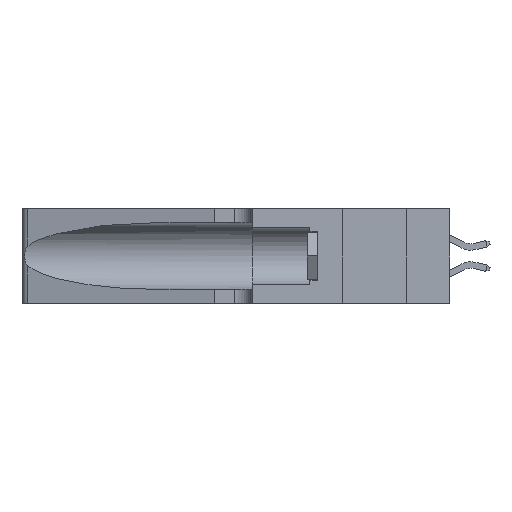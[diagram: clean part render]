
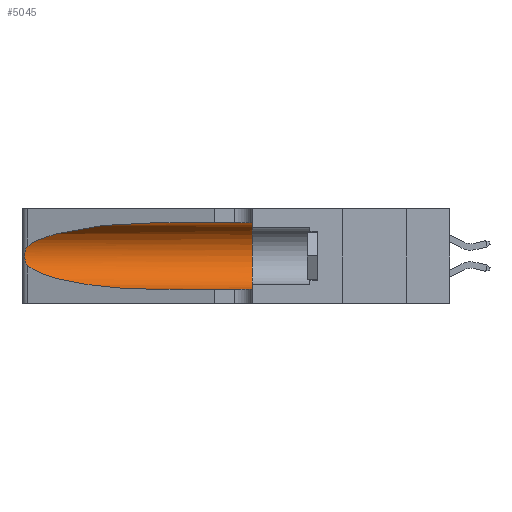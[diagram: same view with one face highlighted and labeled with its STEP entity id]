
A CAD part, left-side view. The second image highlights one B-rep face of the part: STEP entity #5045.
In plain terms, the highlighted cylindrical face has radius 3.308 mm (diameter 6.617 mm), a partial arc.
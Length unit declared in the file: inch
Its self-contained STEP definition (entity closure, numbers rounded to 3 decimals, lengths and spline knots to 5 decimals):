
#160 = CARTESIAN_POINT ( 'NONE',  ( 0.1305, 0.35, 0.31525 ) ) ;
#333 = CARTESIAN_POINT ( 'NONE',  ( 0.26018, 1.23835, 0.19895 ) ) ;
#399 = CARTESIAN_POINT ( 'NONE',  ( 0.25639, 1.23184, 0.21858 ) ) ;
#456 = CARTESIAN_POINT ( 'NONE',  ( 0.25787, 1.23484, 0.2124 ) ) ;
#537 = LINE ( 'NONE', #8476, #4143 ) ;
#1310 = CARTESIAN_POINT ( 'NONE',  ( 0.1305, 0.35, 0.05475 ) ) ;
#1319 = ORIENTED_EDGE ( 'NONE', *, *, #14419, .F. ) ;
#1441 = CARTESIAN_POINT ( 'NONE',  ( 0.1305, 1.61858, 0.31525 ) ) ;
#1626 = ORIENTED_EDGE ( 'NONE', *, *, #3956, .T. ) ;
#1794 = CARTESIAN_POINT ( 'NONE',  ( 0.25555, 1.22993, 0.14849 ) ) ;
#1952 = CARTESIAN_POINT ( 'NONE',  ( 0.18966, 0.96281, 0.05475 ) ) ;
#2091 = VERTEX_POINT ( 'NONE', #4571 ) ;
#3380 = AXIS2_PLACEMENT_3D ( 'NONE', #12026, #4326, #12158 ) ;
#3400 = CIRCLE ( 'NONE', #17091, 0.13025 ) ;
#3585 = DIRECTION ( 'NONE',  ( 0., -1., 0. ) ) ;
#3841 = DIRECTION ( 'NONE',  ( 0., 1., 0. ) ) ;
#3956 = EDGE_CURVE ( 'NONE', #15548, #9490, #14562, .T. ) ;
#4005 = CARTESIAN_POINT ( 'NONE',  ( 0.18966, 0.96281, 0.31525 ) ) ;
#4143 = VECTOR ( 'NONE', #3585, 39.37008 ) ;
#4166 = LINE ( 'NONE', #1441, #7033 ) ;
#4326 = DIRECTION ( 'NONE',  ( 0., -1., 0. ) ) ;
#4384 = EDGE_CURVE ( 'NONE', #12769, #15548, #13353, .T. ) ;
#4571 = CARTESIAN_POINT ( 'NONE',  ( 0.1305, 0.72297, 0.31525 ) ) ;
#4754 =( BOUNDED_CURVE ( )  B_SPLINE_CURVE ( 3, ( #10087, #4005, #13097, #7075 ),
 .UNSPECIFIED., .F., .T. ) 
 B_SPLINE_CURVE_WITH_KNOTS ( ( 4, 4 ),
 ( 1.5708, 2.84003 ),
 .UNSPECIFIED. ) 
 CURVE ( )  GEOMETRIC_REPRESENTATION_ITEM ( )  RATIONAL_B_SPLINE_CURVE ( ( 1., 0.87, 0.87, 1. ) ) 
 REPRESENTATION_ITEM ( '' )  );
#5045 = ADVANCED_FACE ( 'NONE', ( #7162 ), #16280, .F. ) ;
#5279 = EDGE_CURVE ( 'NONE', #2091, #12769, #4754, .T. ) ;
#5380 = DIRECTION ( 'NONE',  ( 0., 0., 1. ) ) ;
#6236 = CARTESIAN_POINT ( 'NONE',  ( 0.25487, 1.22718, 0.22369 ) ) ;
#6486 = CARTESIAN_POINT ( 'NONE',  ( 0.26017, 1.23833, 0.17102 ) ) ;
#7033 = VECTOR ( 'NONE', #7610, 39.37008 ) ;
#7075 = CARTESIAN_POINT ( 'NONE',  ( 0.25487, 1.22718, 0.22369 ) ) ;
#7162 = FACE_OUTER_BOUND ( 'NONE', #13725, .T. ) ;
#7224 = EDGE_CURVE ( 'NONE', #9490, #12020, #537, .T. ) ;
#7599 = ORIENTED_EDGE ( 'NONE', *, *, #5279, .T. ) ;
#7610 = DIRECTION ( 'NONE',  ( 0., -1., 0. ) ) ;
#7881 = CARTESIAN_POINT ( 'NONE',  ( 0.25639, 1.23186, 0.15144 ) ) ;
#8476 = CARTESIAN_POINT ( 'NONE',  ( 0.1305, 1.61858, 0.05475 ) ) ;
#9490 = VERTEX_POINT ( 'NONE', #17009 ) ;
#9787 = CARTESIAN_POINT ( 'NONE',  ( 0.2373, 1.15595, 0.08982 ) ) ;
#10087 = CARTESIAN_POINT ( 'NONE',  ( 0.1305, 0.72297, 0.31525 ) ) ;
#11023 = CARTESIAN_POINT ( 'NONE',  ( 0.25856, 1.23593, 0.16098 ) ) ;
#11125 = CARTESIAN_POINT ( 'NONE',  ( 0.1305, 0.72297, 0.05475 ) ) ;
#12020 = VERTEX_POINT ( 'NONE', #1310 ) ;
#12026 = CARTESIAN_POINT ( 'NONE',  ( 0.1305, 1.61858, 0.185 ) ) ;
#12158 = DIRECTION ( 'NONE',  ( 0., 0., -1. ) ) ;
#12270 = VERTEX_POINT ( 'NONE', #160 ) ;
#12389 = CARTESIAN_POINT ( 'NONE',  ( 0.26075, 1.23896, 0.178 ) ) ;
#12453 = CARTESIAN_POINT ( 'NONE',  ( 0.25487, 1.22718, 0.14631 ) ) ;
#12581 = CARTESIAN_POINT ( 'NONE',  ( 0.25789, 1.23486, 0.15765 ) ) ;
#12769 = VERTEX_POINT ( 'NONE', #6236 ) ;
#13097 = CARTESIAN_POINT ( 'NONE',  ( 0.2373, 1.15595, 0.28018 ) ) ;
#13353 = B_SPLINE_CURVE_WITH_KNOTS ( 'NONE', 3,
 ( #18504, #15591, #399, #456, #18695, #333, #15669, #12389, #6486, #11023, #12581, #7881, #1794, #12453 ),
 .UNSPECIFIED., .F., .F.,
 ( 4, 2, 2, 2, 2, 2, 4 ),
 ( 0., 0.00027, 0.00053, 0.00107, 0.0016, 0.00187, 0.00214 ),
 .UNSPECIFIED. ) ;
#13725 = EDGE_LOOP ( 'NONE', ( #7599, #18882, #1626, #18630, #1319, #15593 ) ) ;
#13955 = EDGE_CURVE ( 'NONE', #2091, #12270, #4166, .T. ) ;
#14419 = EDGE_CURVE ( 'NONE', #12270, #12020, #3400, .T. ) ;
#14562 =( BOUNDED_CURVE ( )  B_SPLINE_CURVE ( 3, ( #18917, #9787, #1952, #11125 ),
 .UNSPECIFIED., .F., .T. ) 
 B_SPLINE_CURVE_WITH_KNOTS ( ( 4, 4 ),
 ( 3.44316, 4.71239 ),
 .UNSPECIFIED. ) 
 CURVE ( )  GEOMETRIC_REPRESENTATION_ITEM ( )  RATIONAL_B_SPLINE_CURVE ( ( 1., 0.87, 0.87, 1. ) ) 
 REPRESENTATION_ITEM ( '' )  );
#15548 = VERTEX_POINT ( 'NONE', #16920 ) ;
#15591 = CARTESIAN_POINT ( 'NONE',  ( 0.25555, 1.22994, 0.2215 ) ) ;
#15593 = ORIENTED_EDGE ( 'NONE', *, *, #13955, .F. ) ;
#15669 = CARTESIAN_POINT ( 'NONE',  ( 0.26075, 1.23896, 0.19203 ) ) ;
#15973 = CARTESIAN_POINT ( 'NONE',  ( 0.1305, 0.35, 0.185 ) ) ;
#16280 = CYLINDRICAL_SURFACE ( 'NONE', #3380, 0.13025 ) ;
#16920 = CARTESIAN_POINT ( 'NONE',  ( 0.25487, 1.22718, 0.14631 ) ) ;
#17009 = CARTESIAN_POINT ( 'NONE',  ( 0.1305, 0.72297, 0.05475 ) ) ;
#17091 = AXIS2_PLACEMENT_3D ( 'NONE', #15973, #3841, #5380 ) ;
#18504 = CARTESIAN_POINT ( 'NONE',  ( 0.25487, 1.22718, 0.22369 ) ) ;
#18630 = ORIENTED_EDGE ( 'NONE', *, *, #7224, .T. ) ;
#18695 = CARTESIAN_POINT ( 'NONE',  ( 0.25854, 1.2359, 0.20912 ) ) ;
#18882 = ORIENTED_EDGE ( 'NONE', *, *, #4384, .T. ) ;
#18917 = CARTESIAN_POINT ( 'NONE',  ( 0.25487, 1.22718, 0.14631 ) ) ;
